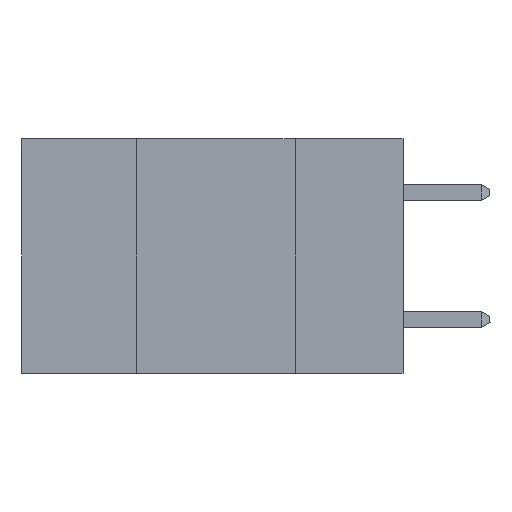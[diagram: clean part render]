
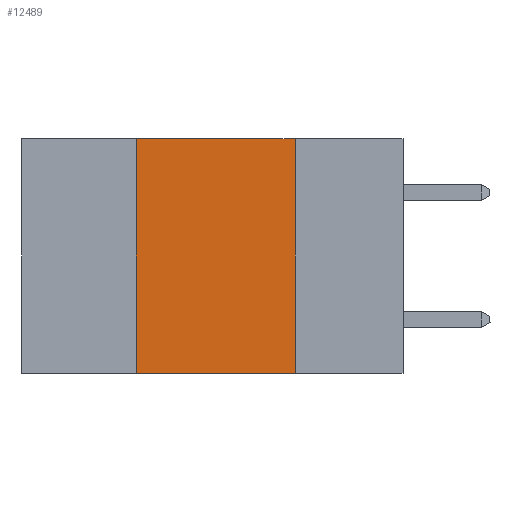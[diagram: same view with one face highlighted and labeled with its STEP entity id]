
A CAD part, left-side view. The second image highlights one B-rep face of the part: STEP entity #12489.
In plain terms, the highlighted planar face has unit normal (-1, 0, 0).
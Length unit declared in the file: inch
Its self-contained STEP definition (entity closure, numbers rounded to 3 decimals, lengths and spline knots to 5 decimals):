
#454 = EDGE_CURVE ( 'NONE', #4707, #11443, #19027, .T. ) ;
#1004 = CARTESIAN_POINT ( 'NONE',  ( 0., 0.6, 0. ) ) ;
#1019 = LINE ( 'NONE', #6678, #6128 ) ;
#1207 = DIRECTION ( 'NONE',  ( 1., 0., 0. ) ) ;
#2449 = LINE ( 'NONE', #4522, #4242 ) ;
#2498 = EDGE_LOOP ( 'NONE', ( #5076, #7242, #10749, #18297 ) ) ;
#2769 = CARTESIAN_POINT ( 'NONE',  ( 0., 0.42, 0. ) ) ;
#3316 = EDGE_CURVE ( 'NONE', #13199, #4707, #19568, .T. ) ;
#4242 = VECTOR ( 'NONE', #4642, 39.37008 ) ;
#4522 = CARTESIAN_POINT ( 'NONE',  ( 0., 0.6, -0.37 ) ) ;
#4636 = EDGE_CURVE ( 'NONE', #15563, #11443, #2449, .T. ) ;
#4642 = DIRECTION ( 'NONE',  ( 0., -1., 0. ) ) ;
#4707 = VERTEX_POINT ( 'NONE', #4803 ) ;
#4803 = CARTESIAN_POINT ( 'NONE',  ( 0., 0.17, 0. ) ) ;
#5076 = ORIENTED_EDGE ( 'NONE', *, *, #454, .F. ) ;
#5284 = DIRECTION ( 'NONE',  ( 0., 0., 1. ) ) ;
#6128 = VECTOR ( 'NONE', #5284, 39.37008 ) ;
#6678 = CARTESIAN_POINT ( 'NONE',  ( 0., 0.42, 0. ) ) ;
#6769 = CARTESIAN_POINT ( 'NONE',  ( 0., 0.17, 0. ) ) ;
#7131 = CARTESIAN_POINT ( 'NONE',  ( 0., 0.17, -0.37 ) ) ;
#7242 = ORIENTED_EDGE ( 'NONE', *, *, #3316, .F. ) ;
#8422 = DIRECTION ( 'NONE',  ( 0., 0., -1. ) ) ;
#9224 = CARTESIAN_POINT ( 'NONE',  ( 0., 0.42, -0.37 ) ) ;
#9661 = VECTOR ( 'NONE', #8422, 39.37008 ) ;
#10749 = ORIENTED_EDGE ( 'NONE', *, *, #20631, .F. ) ;
#11443 = VERTEX_POINT ( 'NONE', #7131 ) ;
#12489 = ADVANCED_FACE ( 'NONE', ( #16059 ), #17610, .F. ) ;
#13199 = VERTEX_POINT ( 'NONE', #2769 ) ;
#14223 = DIRECTION ( 'NONE',  ( 0., -1., 0. ) ) ;
#15563 = VERTEX_POINT ( 'NONE', #9224 ) ;
#16059 = FACE_OUTER_BOUND ( 'NONE', #2498, .T. ) ;
#17610 = PLANE ( 'NONE',  #20348 ) ;
#18297 = ORIENTED_EDGE ( 'NONE', *, *, #4636, .T. ) ;
#19027 = LINE ( 'NONE', #6769, #9661 ) ;
#19515 = CARTESIAN_POINT ( 'NONE',  ( 0., 0.6, 0. ) ) ;
#19568 = LINE ( 'NONE', #19515, #20626 ) ;
#20348 = AXIS2_PLACEMENT_3D ( 'NONE', #1004, #1207, #21093 ) ;
#20626 = VECTOR ( 'NONE', #14223, 39.37008 ) ;
#20631 = EDGE_CURVE ( 'NONE', #15563, #13199, #1019, .T. ) ;
#21093 = DIRECTION ( 'NONE',  ( 0., 0., -1. ) ) ;
